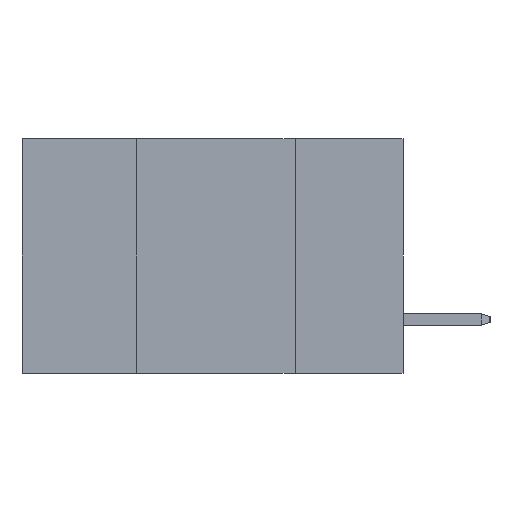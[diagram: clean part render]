
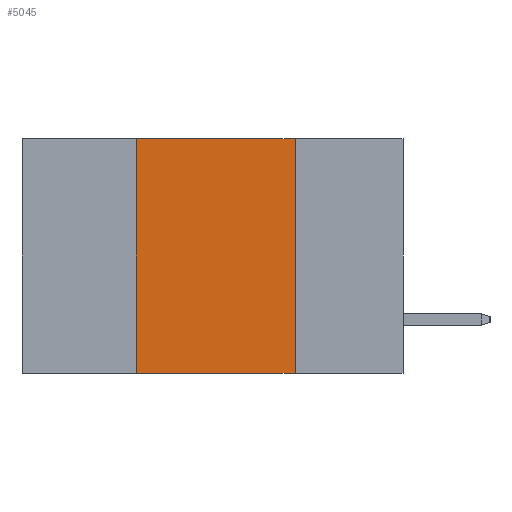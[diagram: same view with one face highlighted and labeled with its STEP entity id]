
A CAD part, left-side view. The second image highlights one B-rep face of the part: STEP entity #5045.
In plain terms, the highlighted planar face has unit normal (-1, 0, 0).
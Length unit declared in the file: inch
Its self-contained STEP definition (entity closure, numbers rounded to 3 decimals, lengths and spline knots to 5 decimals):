
#699 = CARTESIAN_POINT ( 'NONE',  ( 0., 0.6, 0. ) ) ;
#1026 = CARTESIAN_POINT ( 'NONE',  ( 0., 0.6, -0.37 ) ) ;
#1137 = LINE ( 'NONE', #10796, #10270 ) ;
#1414 = EDGE_CURVE ( 'NONE', #8243, #5946, #4103, .T. ) ;
#1580 = VECTOR ( 'NONE', #10610, 39.37008 ) ;
#1969 = EDGE_CURVE ( 'NONE', #11865, #6227, #5226, .T. ) ;
#2255 = CARTESIAN_POINT ( 'NONE',  ( 0., 0.42, 0. ) ) ;
#2993 = EDGE_CURVE ( 'NONE', #8243, #11865, #12518, .T. ) ;
#4103 = LINE ( 'NONE', #1026, #11246 ) ;
#4605 = DIRECTION ( 'NONE',  ( 0., 0., -1. ) ) ;
#4641 = AXIS2_PLACEMENT_3D ( 'NONE', #699, #9455, #4605 ) ;
#4845 = ORIENTED_EDGE ( 'NONE', *, *, #1414, .T. ) ;
#5045 = ADVANCED_FACE ( 'NONE', ( #9524 ), #12455, .F. ) ;
#5129 = CARTESIAN_POINT ( 'NONE',  ( 0., 0.42, -0.37 ) ) ;
#5226 = LINE ( 'NONE', #11938, #11844 ) ;
#5335 = CARTESIAN_POINT ( 'NONE',  ( 0., 0.17, -0.37 ) ) ;
#5820 = ORIENTED_EDGE ( 'NONE', *, *, #12594, .F. ) ;
#5946 = VERTEX_POINT ( 'NONE', #5335 ) ;
#6227 = VERTEX_POINT ( 'NONE', #9868 ) ;
#6963 = EDGE_LOOP ( 'NONE', ( #5820, #11223, #12383, #4845 ) ) ;
#7910 = DIRECTION ( 'NONE',  ( 0., 0., -1. ) ) ;
#7974 = DIRECTION ( 'NONE',  ( 0., -1., 0. ) ) ;
#8243 = VERTEX_POINT ( 'NONE', #5129 ) ;
#9455 = DIRECTION ( 'NONE',  ( 1., 0., 0. ) ) ;
#9524 = FACE_OUTER_BOUND ( 'NONE', #6963, .T. ) ;
#9845 = DIRECTION ( 'NONE',  ( 0., -1., 0. ) ) ;
#9868 = CARTESIAN_POINT ( 'NONE',  ( 0., 0.17, 0. ) ) ;
#10270 = VECTOR ( 'NONE', #7910, 39.37008 ) ;
#10610 = DIRECTION ( 'NONE',  ( 0., 0., 1. ) ) ;
#10796 = CARTESIAN_POINT ( 'NONE',  ( 0., 0.17, 0. ) ) ;
#11223 = ORIENTED_EDGE ( 'NONE', *, *, #1969, .F. ) ;
#11246 = VECTOR ( 'NONE', #9845, 39.37008 ) ;
#11844 = VECTOR ( 'NONE', #7974, 39.37008 ) ;
#11865 = VERTEX_POINT ( 'NONE', #2255 ) ;
#11938 = CARTESIAN_POINT ( 'NONE',  ( 0., 0.6, 0. ) ) ;
#12322 = CARTESIAN_POINT ( 'NONE',  ( 0., 0.42, 0. ) ) ;
#12383 = ORIENTED_EDGE ( 'NONE', *, *, #2993, .F. ) ;
#12455 = PLANE ( 'NONE',  #4641 ) ;
#12518 = LINE ( 'NONE', #12322, #1580 ) ;
#12594 = EDGE_CURVE ( 'NONE', #6227, #5946, #1137, .T. ) ;
